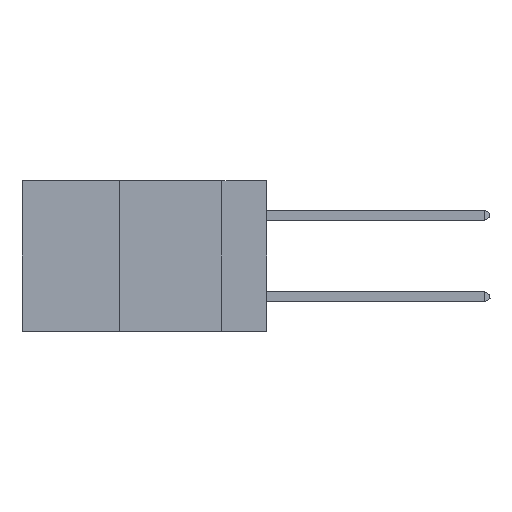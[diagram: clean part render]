
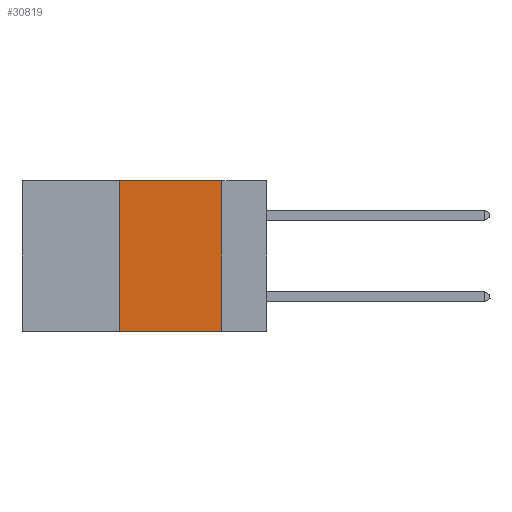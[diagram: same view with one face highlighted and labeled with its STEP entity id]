
A CAD part, left-side view. The second image highlights one B-rep face of the part: STEP entity #30819.
In plain terms, the highlighted planar face has unit normal (-1, 0, 0).
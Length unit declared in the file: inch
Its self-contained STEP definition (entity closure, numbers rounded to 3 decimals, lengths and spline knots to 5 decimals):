
#101 = PLANE ( 'NONE',  #2676 ) ;
#191 = VERTEX_POINT ( 'NONE', #27407 ) ;
#1477 = EDGE_CURVE ( 'NONE', #28152, #32067, #16197, .T. ) ;
#2396 = CARTESIAN_POINT ( 'NONE',  ( 0., 0.6, 0. ) ) ;
#2517 = VECTOR ( 'NONE', #6128, 39.37008 ) ;
#2676 = AXIS2_PLACEMENT_3D ( 'NONE', #2396, #20917, #26066 ) ;
#3818 = EDGE_CURVE ( 'NONE', #32067, #191, #33201, .T. ) ;
#4759 = CARTESIAN_POINT ( 'NONE',  ( 0., 0.36, -0.37 ) ) ;
#5162 = CARTESIAN_POINT ( 'NONE',  ( 0., 0.6, 0. ) ) ;
#5648 = VECTOR ( 'NONE', #10939, 39.37008 ) ;
#6128 = DIRECTION ( 'NONE',  ( 0., -1., 0. ) ) ;
#7386 = LINE ( 'NONE', #13512, #2517 ) ;
#10939 = DIRECTION ( 'NONE',  ( 0., 0., 1. ) ) ;
#12241 = LINE ( 'NONE', #22159, #22400 ) ;
#12699 = CARTESIAN_POINT ( 'NONE',  ( 0., 0.11, -0.37 ) ) ;
#13512 = CARTESIAN_POINT ( 'NONE',  ( 0., 0.6, -0.37 ) ) ;
#14281 = EDGE_LOOP ( 'NONE', ( #31318, #31057, #18263, #18564 ) ) ;
#15999 = VERTEX_POINT ( 'NONE', #12699 ) ;
#16197 = LINE ( 'NONE', #23935, #5648 ) ;
#18263 = ORIENTED_EDGE ( 'NONE', *, *, #1477, .F. ) ;
#18564 = ORIENTED_EDGE ( 'NONE', *, *, #28950, .T. ) ;
#19032 = EDGE_CURVE ( 'NONE', #191, #15999, #12241, .T. ) ;
#19370 = VECTOR ( 'NONE', #20495, 39.37008 ) ;
#19642 = DIRECTION ( 'NONE',  ( 0., 0., -1. ) ) ;
#20495 = DIRECTION ( 'NONE',  ( 0., -1., 0. ) ) ;
#20917 = DIRECTION ( 'NONE',  ( 1., 0., 0. ) ) ;
#22159 = CARTESIAN_POINT ( 'NONE',  ( 0., 0.11, 0. ) ) ;
#22400 = VECTOR ( 'NONE', #19642, 39.37008 ) ;
#23935 = CARTESIAN_POINT ( 'NONE',  ( 0., 0.36, 0. ) ) ;
#25157 = CARTESIAN_POINT ( 'NONE',  ( 0., 0.36, 0. ) ) ;
#26066 = DIRECTION ( 'NONE',  ( 0., 0., -1. ) ) ;
#27407 = CARTESIAN_POINT ( 'NONE',  ( 0., 0.11, 0. ) ) ;
#28152 = VERTEX_POINT ( 'NONE', #4759 ) ;
#28950 = EDGE_CURVE ( 'NONE', #28152, #15999, #7386, .T. ) ;
#29195 = FACE_OUTER_BOUND ( 'NONE', #14281, .T. ) ;
#30819 = ADVANCED_FACE ( 'NONE', ( #29195 ), #101, .F. ) ;
#31057 = ORIENTED_EDGE ( 'NONE', *, *, #3818, .F. ) ;
#31318 = ORIENTED_EDGE ( 'NONE', *, *, #19032, .F. ) ;
#32067 = VERTEX_POINT ( 'NONE', #25157 ) ;
#33201 = LINE ( 'NONE', #5162, #19370 ) ;
